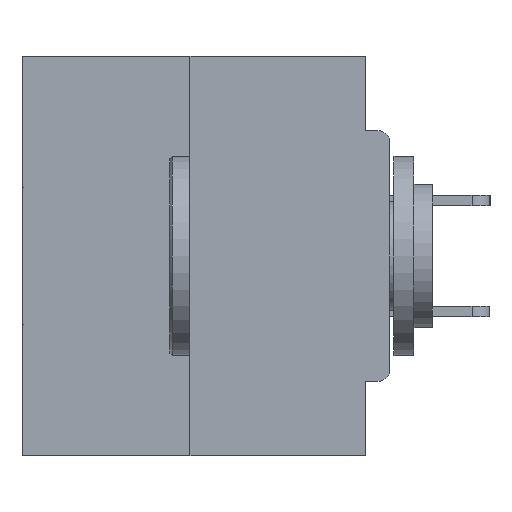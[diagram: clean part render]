
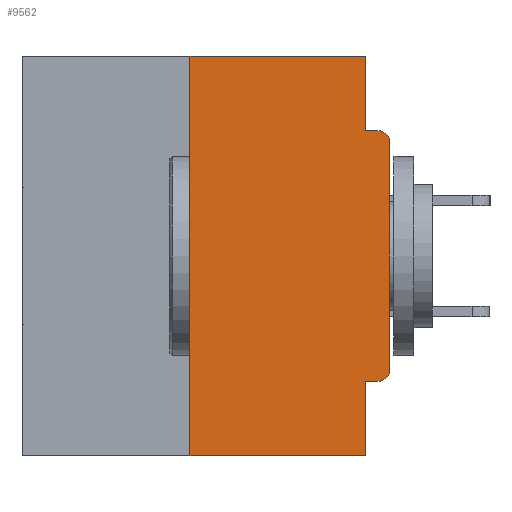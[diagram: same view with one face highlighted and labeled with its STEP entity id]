
A CAD part, left-side view. The second image highlights one B-rep face of the part: STEP entity #9562.
In plain terms, the highlighted planar face has unit normal (-1, 0, 0).
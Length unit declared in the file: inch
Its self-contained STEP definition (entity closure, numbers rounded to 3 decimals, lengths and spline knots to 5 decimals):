
#391 = ORIENTED_EDGE ( 'NONE', *, *, #19455, .T. ) ;
#629 = VERTEX_POINT ( 'NONE', #3096 ) ;
#1213 = CARTESIAN_POINT ( 'NONE',  ( 0., 0.031, -0.4065 ) ) ;
#1237 = VERTEX_POINT ( 'NONE', #15925 ) ;
#1653 = LINE ( 'NONE', #30256, #37607 ) ;
#2470 = LINE ( 'NONE', #38710, #39365 ) ;
#2489 = EDGE_CURVE ( 'NONE', #21487, #3007, #23337, .T. ) ;
#2569 = EDGE_CURVE ( 'NONE', #19788, #8071, #18527, .T. ) ;
#2782 = VECTOR ( 'NONE', #30035, 39.37008 ) ;
#3007 = VERTEX_POINT ( 'NONE', #36040 ) ;
#3096 = CARTESIAN_POINT ( 'NONE',  ( 0., 0.031, -0.5 ) ) ;
#3961 = AXIS2_PLACEMENT_3D ( 'NONE', #15999, #13327, #31841 ) ;
#4249 = EDGE_CURVE ( 'NONE', #22540, #629, #1653, .T. ) ;
#4464 = PLANE ( 'NONE',  #14883 ) ;
#4811 = VECTOR ( 'NONE', #7772, 39.37008 ) ;
#5412 = CARTESIAN_POINT ( 'NONE',  ( 0., 0., -0.3915 ) ) ;
#6147 = EDGE_CURVE ( 'NONE', #8071, #629, #13419, .T. ) ;
#6213 = ORIENTED_EDGE ( 'NONE', *, *, #21341, .T. ) ;
#6411 = ORIENTED_EDGE ( 'NONE', *, *, #2489, .T. ) ;
#7772 = DIRECTION ( 'NONE',  ( 0., -1., 0. ) ) ;
#8071 = VERTEX_POINT ( 'NONE', #1213 ) ;
#8582 = CARTESIAN_POINT ( 'NONE',  ( 0., 0., -0.4065 ) ) ;
#9111 = VECTOR ( 'NONE', #19533, 39.37008 ) ;
#9562 = ADVANCED_FACE ( 'NONE', ( #23323 ), #4464, .F. ) ;
#10380 = CARTESIAN_POINT ( 'NONE',  ( 0., 0.46, 0. ) ) ;
#10524 = CARTESIAN_POINT ( 'NONE',  ( 0., 0.031, -0.5 ) ) ;
#11058 = DIRECTION ( 'NONE',  ( 0., 0., -1. ) ) ;
#11167 = VERTEX_POINT ( 'NONE', #15637 ) ;
#13327 = DIRECTION ( 'NONE',  ( -1., 0., 0. ) ) ;
#13419 = LINE ( 'NONE', #10524, #34577 ) ;
#14883 = AXIS2_PLACEMENT_3D ( 'NONE', #10380, #19435, #35148 ) ;
#15579 = EDGE_LOOP ( 'NONE', ( #19898, #18005, #24364, #28973, #38074, #6213, #391, #6411, #21942, #30611 ) ) ;
#15637 = CARTESIAN_POINT ( 'NONE',  ( 0., 0.25, 0. ) ) ;
#15925 = CARTESIAN_POINT ( 'NONE',  ( 0., 0.031, 0. ) ) ;
#15999 = CARTESIAN_POINT ( 'NONE',  ( 0., 0.015, -0.3915 ) ) ;
#16665 = AXIS2_PLACEMENT_3D ( 'NONE', #32713, #17383, #23443 ) ;
#17344 = DIRECTION ( 'NONE',  ( 0., 0., 1. ) ) ;
#17383 = DIRECTION ( 'NONE',  ( -1., 0., 0. ) ) ;
#17535 = CARTESIAN_POINT ( 'NONE',  ( 0., 0.015, -0.4065 ) ) ;
#17888 = CARTESIAN_POINT ( 'NONE',  ( 0., 0.031, -0.0935 ) ) ;
#18005 = ORIENTED_EDGE ( 'NONE', *, *, #31653, .F. ) ;
#18527 = LINE ( 'NONE', #8582, #2782 ) ;
#19435 = DIRECTION ( 'NONE',  ( 1., 0., 0. ) ) ;
#19455 = EDGE_CURVE ( 'NONE', #23125, #21487, #31795, .T. ) ;
#19533 = DIRECTION ( 'NONE',  ( 0., -1., 0. ) ) ;
#19788 = VERTEX_POINT ( 'NONE', #17535 ) ;
#19898 = ORIENTED_EDGE ( 'NONE', *, *, #32060, .F. ) ;
#20248 = VECTOR ( 'NONE', #17344, 39.37008 ) ;
#20270 = VECTOR ( 'NONE', #29242, 39.37008 ) ;
#21341 = EDGE_CURVE ( 'NONE', #19788, #23125, #22728, .T. ) ;
#21487 = VERTEX_POINT ( 'NONE', #38259 ) ;
#21942 = ORIENTED_EDGE ( 'NONE', *, *, #23715, .F. ) ;
#22045 = EDGE_CURVE ( 'NONE', #1237, #35244, #23167, .T. ) ;
#22540 = VERTEX_POINT ( 'NONE', #24372 ) ;
#22632 = CARTESIAN_POINT ( 'NONE',  ( 0., 0.031, 0. ) ) ;
#22728 = CIRCLE ( 'NONE', #3961, 0.015 ) ;
#23125 = VERTEX_POINT ( 'NONE', #5412 ) ;
#23167 = LINE ( 'NONE', #22632, #20270 ) ;
#23323 = FACE_OUTER_BOUND ( 'NONE', #15579, .T. ) ;
#23337 = CIRCLE ( 'NONE', #16665, 0.015 ) ;
#23443 = DIRECTION ( 'NONE',  ( 0., 0., -1. ) ) ;
#23715 = EDGE_CURVE ( 'NONE', #35244, #3007, #38371, .T. ) ;
#23805 = CARTESIAN_POINT ( 'NONE',  ( 0., 0., 0. ) ) ;
#24364 = ORIENTED_EDGE ( 'NONE', *, *, #4249, .T. ) ;
#24372 = CARTESIAN_POINT ( 'NONE',  ( 0., 0.25, -0.5 ) ) ;
#26254 = DIRECTION ( 'NONE',  ( 0., 0., 1. ) ) ;
#27806 = LINE ( 'NONE', #30182, #9111 ) ;
#28973 = ORIENTED_EDGE ( 'NONE', *, *, #6147, .F. ) ;
#29242 = DIRECTION ( 'NONE',  ( 0., 0., -1. ) ) ;
#30035 = DIRECTION ( 'NONE',  ( 0., 1., 0. ) ) ;
#30182 = CARTESIAN_POINT ( 'NONE',  ( 0., 0.46, 0. ) ) ;
#30256 = CARTESIAN_POINT ( 'NONE',  ( 0., 0.46, -0.5 ) ) ;
#30611 = ORIENTED_EDGE ( 'NONE', *, *, #22045, .F. ) ;
#31653 = EDGE_CURVE ( 'NONE', #22540, #11167, #2470, .T. ) ;
#31795 = LINE ( 'NONE', #23805, #20248 ) ;
#31841 = DIRECTION ( 'NONE',  ( 0., 0., -1. ) ) ;
#32060 = EDGE_CURVE ( 'NONE', #11167, #1237, #27806, .T. ) ;
#32713 = CARTESIAN_POINT ( 'NONE',  ( 0., 0.015, -0.1085 ) ) ;
#34577 = VECTOR ( 'NONE', #11058, 39.37008 ) ;
#35148 = DIRECTION ( 'NONE',  ( 0., 0., -1. ) ) ;
#35244 = VERTEX_POINT ( 'NONE', #17888 ) ;
#35791 = CARTESIAN_POINT ( 'NONE',  ( 0., 0., -0.0935 ) ) ;
#36040 = CARTESIAN_POINT ( 'NONE',  ( 0., 0.015, -0.0935 ) ) ;
#36296 = DIRECTION ( 'NONE',  ( 0., -1., 0. ) ) ;
#37607 = VECTOR ( 'NONE', #36296, 39.37008 ) ;
#38074 = ORIENTED_EDGE ( 'NONE', *, *, #2569, .F. ) ;
#38259 = CARTESIAN_POINT ( 'NONE',  ( 0., 0., -0.1085 ) ) ;
#38371 = LINE ( 'NONE', #35791, #4811 ) ;
#38710 = CARTESIAN_POINT ( 'NONE',  ( 0., 0.25, 0. ) ) ;
#39365 = VECTOR ( 'NONE', #26254, 39.37008 ) ;
